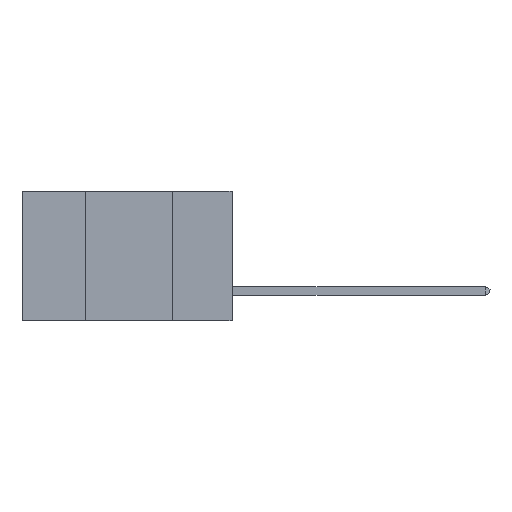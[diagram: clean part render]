
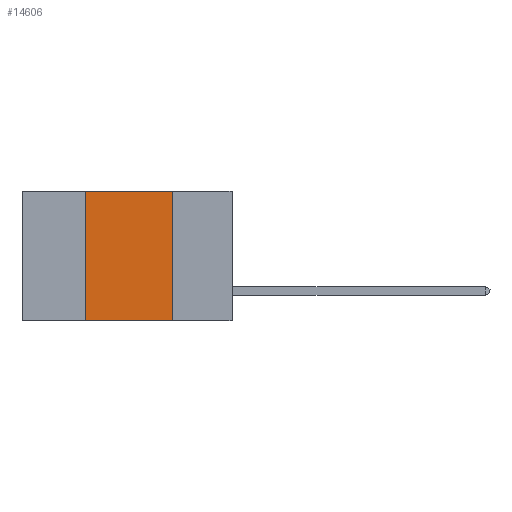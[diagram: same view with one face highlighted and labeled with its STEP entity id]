
A CAD part, left-side view. The second image highlights one B-rep face of the part: STEP entity #14606.
In plain terms, the highlighted planar face has unit normal (-1, 0, 0).
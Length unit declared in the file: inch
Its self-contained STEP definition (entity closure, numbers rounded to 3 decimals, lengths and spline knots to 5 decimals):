
#230 = VERTEX_POINT ( 'NONE', #2748 ) ;
#1292 = CARTESIAN_POINT ( 'NONE',  ( 0., 0.17, -0.37 ) ) ;
#1757 = EDGE_LOOP ( 'NONE', ( #4451, #13675, #5980, #3813 ) ) ;
#2226 = EDGE_CURVE ( 'NONE', #15519, #15125, #11497, .T. ) ;
#2748 = CARTESIAN_POINT ( 'NONE',  ( 0., 0.42, 0. ) ) ;
#3771 = CARTESIAN_POINT ( 'NONE',  ( 0., 0.6, 0. ) ) ;
#3813 = ORIENTED_EDGE ( 'NONE', *, *, #2226, .T. ) ;
#4451 = ORIENTED_EDGE ( 'NONE', *, *, #14907, .F. ) ;
#4775 = CARTESIAN_POINT ( 'NONE',  ( 0., 0.42, 0. ) ) ;
#4841 = LINE ( 'NONE', #6467, #9296 ) ;
#4957 = VECTOR ( 'NONE', #10570, 39.37008 ) ;
#5168 = VECTOR ( 'NONE', #11509, 39.37008 ) ;
#5240 = CARTESIAN_POINT ( 'NONE',  ( 0., 0.17, 0. ) ) ;
#5523 = DIRECTION ( 'NONE',  ( 0., 0., -1. ) ) ;
#5632 = PLANE ( 'NONE',  #8227 ) ;
#5980 = ORIENTED_EDGE ( 'NONE', *, *, #12112, .F. ) ;
#6467 = CARTESIAN_POINT ( 'NONE',  ( 0., 0.17, 0. ) ) ;
#6782 = FACE_OUTER_BOUND ( 'NONE', #1757, .T. ) ;
#7345 = VERTEX_POINT ( 'NONE', #5240 ) ;
#8227 = AXIS2_PLACEMENT_3D ( 'NONE', #8416, #12278, #5523 ) ;
#8416 = CARTESIAN_POINT ( 'NONE',  ( 0., 0.6, 0. ) ) ;
#8556 = LINE ( 'NONE', #3771, #4957 ) ;
#8626 = CARTESIAN_POINT ( 'NONE',  ( 0., 0.6, -0.37 ) ) ;
#8985 = VECTOR ( 'NONE', #14030, 39.37008 ) ;
#9296 = VECTOR ( 'NONE', #17136, 39.37008 ) ;
#10570 = DIRECTION ( 'NONE',  ( 0., -1., 0. ) ) ;
#11497 = LINE ( 'NONE', #8626, #8985 ) ;
#11509 = DIRECTION ( 'NONE',  ( 0., 0., 1. ) ) ;
#11796 = CARTESIAN_POINT ( 'NONE',  ( 0., 0.42, -0.37 ) ) ;
#12109 = LINE ( 'NONE', #4775, #5168 ) ;
#12112 = EDGE_CURVE ( 'NONE', #15519, #230, #12109, .T. ) ;
#12278 = DIRECTION ( 'NONE',  ( 1., 0., 0. ) ) ;
#13675 = ORIENTED_EDGE ( 'NONE', *, *, #17432, .F. ) ;
#14030 = DIRECTION ( 'NONE',  ( 0., -1., 0. ) ) ;
#14606 = ADVANCED_FACE ( 'NONE', ( #6782 ), #5632, .F. ) ;
#14907 = EDGE_CURVE ( 'NONE', #7345, #15125, #4841, .T. ) ;
#15125 = VERTEX_POINT ( 'NONE', #1292 ) ;
#15519 = VERTEX_POINT ( 'NONE', #11796 ) ;
#17136 = DIRECTION ( 'NONE',  ( 0., 0., -1. ) ) ;
#17432 = EDGE_CURVE ( 'NONE', #230, #7345, #8556, .T. ) ;
